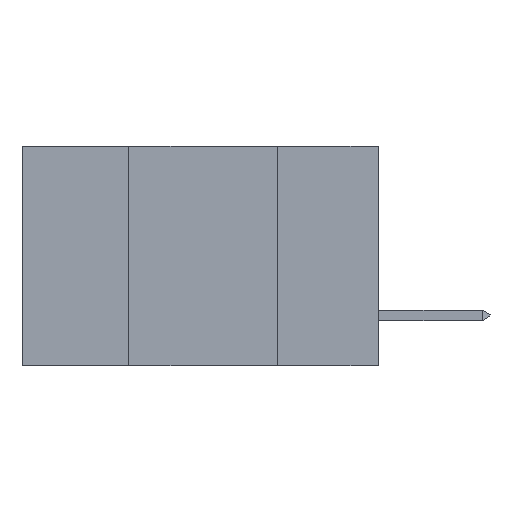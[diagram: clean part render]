
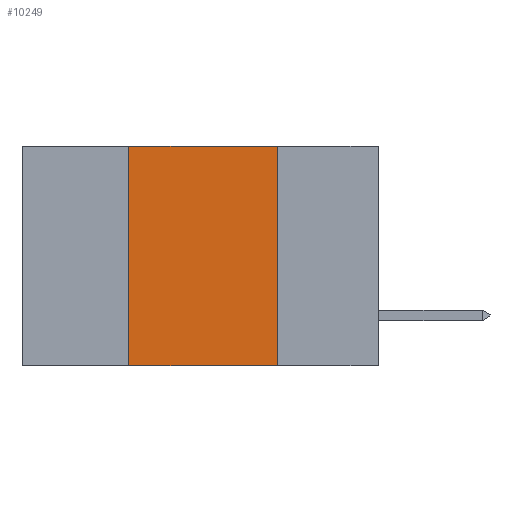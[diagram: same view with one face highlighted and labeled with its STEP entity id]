
A CAD part, left-side view. The second image highlights one B-rep face of the part: STEP entity #10249.
In plain terms, the highlighted planar face has unit normal (-1, 0, 0).
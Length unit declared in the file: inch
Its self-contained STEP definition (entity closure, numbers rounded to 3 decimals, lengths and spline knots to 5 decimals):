
#336 = LINE ( 'NONE', #11625, #5627 ) ;
#1028 = EDGE_CURVE ( 'NONE', #12402, #9568, #9685, .T. ) ;
#1326 = DIRECTION ( 'NONE',  ( 0., 0., -1. ) ) ;
#1516 = ORIENTED_EDGE ( 'NONE', *, *, #1028, .F. ) ;
#1736 = DIRECTION ( 'NONE',  ( 0., 0., -1. ) ) ;
#4366 = CARTESIAN_POINT ( 'NONE',  ( 0., 0.42, -0.37 ) ) ;
#4545 = DIRECTION ( 'NONE',  ( 0., -1., 0. ) ) ;
#4586 = DIRECTION ( 'NONE',  ( 1., 0., 0. ) ) ;
#4883 = VECTOR ( 'NONE', #14504, 39.37008 ) ;
#5097 = DIRECTION ( 'NONE',  ( 0., -1., 0. ) ) ;
#5584 = ORIENTED_EDGE ( 'NONE', *, *, #11426, .T. ) ;
#5621 = VERTEX_POINT ( 'NONE', #10667 ) ;
#5627 = VECTOR ( 'NONE', #1326, 39.37008 ) ;
#5649 = CARTESIAN_POINT ( 'NONE',  ( 0., 0.6, 0. ) ) ;
#6063 = VECTOR ( 'NONE', #4545, 39.37008 ) ;
#6404 = PLANE ( 'NONE',  #7026 ) ;
#7026 = AXIS2_PLACEMENT_3D ( 'NONE', #5649, #4586, #1736 ) ;
#7108 = EDGE_LOOP ( 'NONE', ( #14044, #1516, #10830, #5584 ) ) ;
#8008 = CARTESIAN_POINT ( 'NONE',  ( 0., 0.6, -0.37 ) ) ;
#8544 = VERTEX_POINT ( 'NONE', #11429 ) ;
#8635 = CARTESIAN_POINT ( 'NONE',  ( 0., 0.6, 0. ) ) ;
#8957 = VECTOR ( 'NONE', #5097, 39.37008 ) ;
#9568 = VERTEX_POINT ( 'NONE', #13660 ) ;
#9685 = LINE ( 'NONE', #8635, #8957 ) ;
#10249 = ADVANCED_FACE ( 'NONE', ( #10899 ), #6404, .F. ) ;
#10667 = CARTESIAN_POINT ( 'NONE',  ( 0., 0.42, -0.37 ) ) ;
#10830 = ORIENTED_EDGE ( 'NONE', *, *, #12060, .F. ) ;
#10899 = FACE_OUTER_BOUND ( 'NONE', #7108, .T. ) ;
#11426 = EDGE_CURVE ( 'NONE', #5621, #8544, #12733, .T. ) ;
#11429 = CARTESIAN_POINT ( 'NONE',  ( 0., 0.17, -0.37 ) ) ;
#11625 = CARTESIAN_POINT ( 'NONE',  ( 0., 0.17, -0.37 ) ) ;
#12060 = EDGE_CURVE ( 'NONE', #5621, #12402, #14651, .T. ) ;
#12402 = VERTEX_POINT ( 'NONE', #13417 ) ;
#12733 = LINE ( 'NONE', #8008, #6063 ) ;
#13300 = EDGE_CURVE ( 'NONE', #9568, #8544, #336, .T. ) ;
#13417 = CARTESIAN_POINT ( 'NONE',  ( 0., 0.42, 0. ) ) ;
#13660 = CARTESIAN_POINT ( 'NONE',  ( 0., 0.17, 0. ) ) ;
#14044 = ORIENTED_EDGE ( 'NONE', *, *, #13300, .F. ) ;
#14504 = DIRECTION ( 'NONE',  ( 0., 0., 1. ) ) ;
#14651 = LINE ( 'NONE', #4366, #4883 ) ;
